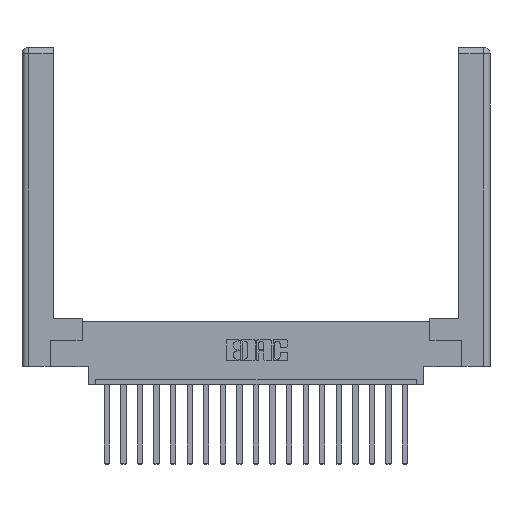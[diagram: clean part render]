
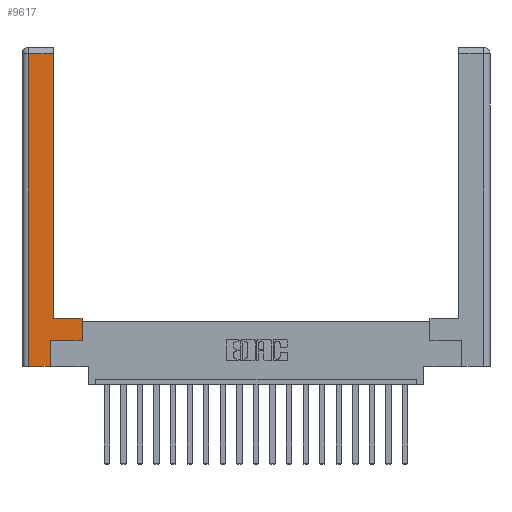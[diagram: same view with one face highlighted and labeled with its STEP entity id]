
A CAD part, top view. The second image highlights one B-rep face of the part: STEP entity #9617.
In plain terms, the highlighted planar face has unit normal (0, 0, 1).
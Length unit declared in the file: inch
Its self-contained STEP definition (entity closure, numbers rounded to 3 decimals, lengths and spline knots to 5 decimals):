
#324 = EDGE_CURVE ( 'NONE', #2974, #17883, #13977, .T. ) ;
#929 = DIRECTION ( 'NONE',  ( 0., 1., 0. ) ) ;
#1812 = LINE ( 'NONE', #12982, #18925 ) ;
#1909 = EDGE_CURVE ( 'NONE', #17862, #2974, #18079, .T. ) ;
#2060 = PLANE ( 'NONE',  #17541 ) ;
#2322 = CARTESIAN_POINT ( 'NONE',  ( 0.295, 2.94, 0. ) ) ;
#2336 = ORIENTED_EDGE ( 'NONE', *, *, #11909, .T. ) ;
#2678 = DIRECTION ( 'NONE',  ( 0., 1., 0. ) ) ;
#2774 = VECTOR ( 'NONE', #2678, 39.37008 ) ;
#2968 = ORIENTED_EDGE ( 'NONE', *, *, #4886, .T. ) ;
#2974 = VERTEX_POINT ( 'NONE', #16592 ) ;
#3643 = DIRECTION ( 'NONE',  ( 0., 0., -1. ) ) ;
#3875 = DIRECTION ( 'NONE',  ( 0., -1., 0. ) ) ;
#4074 = VERTEX_POINT ( 'NONE', #17010 ) ;
#4753 = CARTESIAN_POINT ( 'NONE',  ( 0.0615, 0., 0. ) ) ;
#4865 = ORIENTED_EDGE ( 'NONE', *, *, #324, .T. ) ;
#4886 = EDGE_CURVE ( 'NONE', #7795, #13426, #1812, .T. ) ;
#6538 = DIRECTION ( 'NONE',  ( 0., 1., 0. ) ) ;
#6607 = ORIENTED_EDGE ( 'NONE', *, *, #12971, .T. ) ;
#7244 = CARTESIAN_POINT ( 'NONE',  ( 0.295, 0.45, 0. ) ) ;
#7435 = ORIENTED_EDGE ( 'NONE', *, *, #10809, .T. ) ;
#7795 = VERTEX_POINT ( 'NONE', #16657 ) ;
#8060 = CARTESIAN_POINT ( 'NONE',  ( 0.0615, 0., 0. ) ) ;
#8273 = EDGE_CURVE ( 'NONE', #4074, #7795, #14287, .T. ) ;
#8513 = DIRECTION ( 'NONE',  ( 1., 0., 0. ) ) ;
#8546 = VERTEX_POINT ( 'NONE', #4753 ) ;
#8929 = VECTOR ( 'NONE', #6538, 39.37008 ) ;
#9617 = ADVANCED_FACE ( 'NONE', ( #16822 ), #2060, .F. ) ;
#9937 = ORIENTED_EDGE ( 'NONE', *, *, #8273, .T. ) ;
#10010 = CARTESIAN_POINT ( 'NONE',  ( 0.265, 0.245, 0. ) ) ;
#10154 = CARTESIAN_POINT ( 'NONE',  ( 0.265, 0., 0. ) ) ;
#10211 = ORIENTED_EDGE ( 'NONE', *, *, #1909, .T. ) ;
#10233 = DIRECTION ( 'NONE',  ( -1., 0., 0. ) ) ;
#10375 = CARTESIAN_POINT ( 'NONE',  ( 0.0615, 2.94, 0. ) ) ;
#10809 = EDGE_CURVE ( 'NONE', #17883, #11029, #17228, .T. ) ;
#11029 = VERTEX_POINT ( 'NONE', #10375 ) ;
#11507 = LINE ( 'NONE', #13779, #8929 ) ;
#11909 = EDGE_CURVE ( 'NONE', #13426, #17862, #11507, .T. ) ;
#11986 = DIRECTION ( 'NONE',  ( -1., 0., 0. ) ) ;
#12479 = VECTOR ( 'NONE', #8513, 39.37008 ) ;
#12524 = EDGE_CURVE ( 'NONE', #11029, #8546, #18378, .T. ) ;
#12715 = DIRECTION ( 'NONE',  ( -1., 0., 0. ) ) ;
#12971 = EDGE_CURVE ( 'NONE', #8546, #4074, #14868, .T. ) ;
#12977 = VECTOR ( 'NONE', #11986, 39.37008 ) ;
#12982 = CARTESIAN_POINT ( 'NONE',  ( 0.565, 0.245, 0. ) ) ;
#13355 = VECTOR ( 'NONE', #10233, 39.37008 ) ;
#13426 = VERTEX_POINT ( 'NONE', #16151 ) ;
#13779 = CARTESIAN_POINT ( 'NONE',  ( 0.565, 0.45, 0. ) ) ;
#13977 = LINE ( 'NONE', #16281, #2774 ) ;
#14045 = CARTESIAN_POINT ( 'NONE',  ( 0., 0., 0. ) ) ;
#14287 = LINE ( 'NONE', #10010, #19008 ) ;
#14868 = LINE ( 'NONE', #10154, #12479 ) ;
#15240 = EDGE_LOOP ( 'NONE', ( #4865, #7435, #17596, #6607, #9937, #2968, #2336, #10211 ) ) ;
#15904 = DIRECTION ( 'NONE',  ( 1., 0., 0. ) ) ;
#16151 = CARTESIAN_POINT ( 'NONE',  ( 0.565, 0.245, 0. ) ) ;
#16281 = CARTESIAN_POINT ( 'NONE',  ( 0.295, 3., 0. ) ) ;
#16324 = CARTESIAN_POINT ( 'NONE',  ( 0.0615, 2.94, 0. ) ) ;
#16592 = CARTESIAN_POINT ( 'NONE',  ( 0.295, 0.45, 0. ) ) ;
#16657 = CARTESIAN_POINT ( 'NONE',  ( 0.265, 0.245, 0. ) ) ;
#16822 = FACE_OUTER_BOUND ( 'NONE', #15240, .T. ) ;
#17010 = CARTESIAN_POINT ( 'NONE',  ( 0.265, 0., 0. ) ) ;
#17228 = LINE ( 'NONE', #16324, #12977 ) ;
#17541 = AXIS2_PLACEMENT_3D ( 'NONE', #14045, #3643, #12715 ) ;
#17596 = ORIENTED_EDGE ( 'NONE', *, *, #12524, .T. ) ;
#17862 = VERTEX_POINT ( 'NONE', #18934 ) ;
#17883 = VERTEX_POINT ( 'NONE', #2322 ) ;
#17895 = VECTOR ( 'NONE', #3875, 39.37008 ) ;
#18079 = LINE ( 'NONE', #7244, #13355 ) ;
#18378 = LINE ( 'NONE', #8060, #17895 ) ;
#18925 = VECTOR ( 'NONE', #15904, 39.37008 ) ;
#18934 = CARTESIAN_POINT ( 'NONE',  ( 0.565, 0.45, 0. ) ) ;
#19008 = VECTOR ( 'NONE', #929, 39.37008 ) ;
